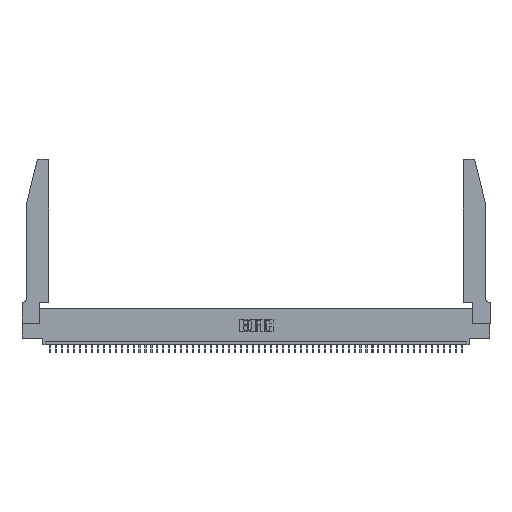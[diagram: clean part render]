
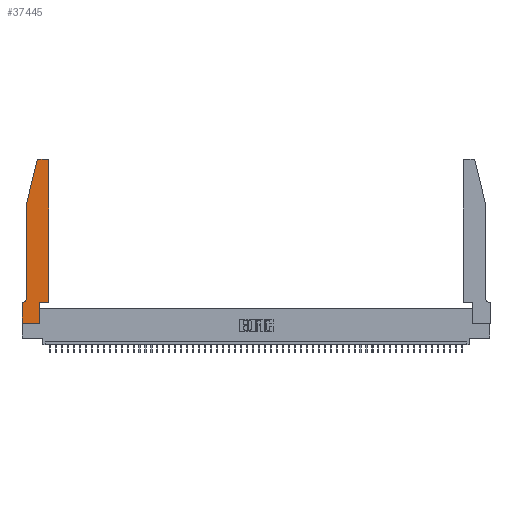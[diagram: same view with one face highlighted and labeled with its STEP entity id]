
A CAD part, top view. The second image highlights one B-rep face of the part: STEP entity #37445.
In plain terms, the highlighted planar face has unit normal (0, 0, 1).
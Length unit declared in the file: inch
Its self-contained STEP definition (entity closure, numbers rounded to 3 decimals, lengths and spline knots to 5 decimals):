
#258 = ORIENTED_EDGE ( 'NONE', *, *, #11909, .T. ) ;
#563 = CARTESIAN_POINT ( 'NONE',  ( 0., 0., 0.37 ) ) ;
#596 = VECTOR ( 'NONE', #46374, 39.37008 ) ;
#936 = VERTEX_POINT ( 'NONE', #29990 ) ;
#1106 = CARTESIAN_POINT ( 'NONE',  ( 0.0755, 2., 0.37 ) ) ;
#1564 = CARTESIAN_POINT ( 'NONE',  ( 0.4505, 0.35, 0.37 ) ) ;
#2447 = CIRCLE ( 'NONE', #44126, 0.03 ) ;
#2887 = VERTEX_POINT ( 'NONE', #3976 ) ;
#3383 = VERTEX_POINT ( 'NONE', #29261 ) ;
#3976 = CARTESIAN_POINT ( 'NONE',  ( 0.4205, 2.75, 0.37 ) ) ;
#4281 = ORIENTED_EDGE ( 'NONE', *, *, #52299, .T. ) ;
#6387 = CARTESIAN_POINT ( 'NONE',  ( 0.0755, 2., 0.37 ) ) ;
#6652 = VECTOR ( 'NONE', #6730, 39.37008 ) ;
#6730 = DIRECTION ( 'NONE',  ( 0., -1., 0. ) ) ;
#6797 = DIRECTION ( 'NONE',  ( 0., 0., 1. ) ) ;
#7917 = DIRECTION ( 'NONE',  ( -1., 0., 0. ) ) ;
#8159 = CARTESIAN_POINT ( 'NONE',  ( 0., 0.35, 0.37 ) ) ;
#8361 = VERTEX_POINT ( 'NONE', #37701 ) ;
#8521 = VECTOR ( 'NONE', #18210, 39.37008 ) ;
#9204 = LINE ( 'NONE', #1564, #8521 ) ;
#9491 = EDGE_CURVE ( 'NONE', #39485, #41257, #18701, .T. ) ;
#9911 = PLANE ( 'NONE',  #30217 ) ;
#10360 = LINE ( 'NONE', #26159, #34873 ) ;
#10808 = CARTESIAN_POINT ( 'NONE',  ( 0.2865, 0.35, 0.37 ) ) ;
#11101 = VECTOR ( 'NONE', #22383, 39.37008 ) ;
#11566 = ORIENTED_EDGE ( 'NONE', *, *, #42108, .T. ) ;
#11909 = EDGE_CURVE ( 'NONE', #45939, #35143, #14349, .T. ) ;
#12085 = AXIS2_PLACEMENT_3D ( 'NONE', #32163, #6797, #15284 ) ;
#12240 = CARTESIAN_POINT ( 'NONE',  ( 0.0055, 0.35, 0.37 ) ) ;
#12874 = VERTEX_POINT ( 'NONE', #18294 ) ;
#12935 = CIRCLE ( 'NONE', #12085, 0.03 ) ;
#14283 = DIRECTION ( 'NONE',  ( 0., 0., 1. ) ) ;
#14349 = LINE ( 'NONE', #17869, #30030 ) ;
#15284 = DIRECTION ( 'NONE',  ( 1., 0., 0. ) ) ;
#16273 = EDGE_LOOP ( 'NONE', ( #22857, #35106, #39636, #48043, #29615, #33045, #4281, #258, #11566, #48635, #43502, #42557 ) ) ;
#17751 = LINE ( 'NONE', #563, #596 ) ;
#17869 = CARTESIAN_POINT ( 'NONE',  ( 0., 0., 0.37 ) ) ;
#18210 = DIRECTION ( 'NONE',  ( 0., 1., 0. ) ) ;
#18294 = CARTESIAN_POINT ( 'NONE',  ( 0.25487, 2.72718, 0.37 ) ) ;
#18701 = CIRCLE ( 'NONE', #34368, 0.07 ) ;
#19754 = EDGE_CURVE ( 'NONE', #25671, #3383, #10360, .T. ) ;
#21953 = LINE ( 'NONE', #6387, #46335 ) ;
#21958 = EDGE_CURVE ( 'NONE', #12874, #46717, #21953, .T. ) ;
#22383 = DIRECTION ( 'NONE',  ( -1., 0., 0. ) ) ;
#22506 = DIRECTION ( 'NONE',  ( 1., 0., 0. ) ) ;
#22708 = CARTESIAN_POINT ( 'NONE',  ( 0.0055, 0.42, 0.37 ) ) ;
#22857 = ORIENTED_EDGE ( 'NONE', *, *, #52084, .T. ) ;
#23957 = EDGE_CURVE ( 'NONE', #46717, #39485, #47458, .T. ) ;
#25671 = VERTEX_POINT ( 'NONE', #10808 ) ;
#26159 = CARTESIAN_POINT ( 'NONE',  ( 0.4505, 0.35, 0.37 ) ) ;
#27401 = CARTESIAN_POINT ( 'NONE',  ( 0.284, 2.72, 0.37 ) ) ;
#28149 = VERTEX_POINT ( 'NONE', #8159 ) ;
#28371 = DIRECTION ( 'NONE',  ( 0., 0., -1. ) ) ;
#29261 = CARTESIAN_POINT ( 'NONE',  ( 0.4505, 0.35, 0.37 ) ) ;
#29615 = ORIENTED_EDGE ( 'NONE', *, *, #9491, .T. ) ;
#29990 = CARTESIAN_POINT ( 'NONE',  ( 0.4505, 2.72, 0.37 ) ) ;
#30030 = VECTOR ( 'NONE', #22506, 39.37008 ) ;
#30208 = CARTESIAN_POINT ( 'NONE',  ( 0.0755, 0.42, 0.37 ) ) ;
#30217 = AXIS2_PLACEMENT_3D ( 'NONE', #43148, #14283, #30877 ) ;
#30592 = CARTESIAN_POINT ( 'NONE',  ( 0., 0., 0.37 ) ) ;
#30810 = LINE ( 'NONE', #51836, #11101 ) ;
#30877 = DIRECTION ( 'NONE',  ( 1., 0., 0. ) ) ;
#30942 = CARTESIAN_POINT ( 'NONE',  ( 0.2865, 0.35, 0.37 ) ) ;
#31762 = DIRECTION ( 'NONE',  ( 1., 0., 0. ) ) ;
#32163 = CARTESIAN_POINT ( 'NONE',  ( 0.4205, 2.72, 0.37 ) ) ;
#32829 = VECTOR ( 'NONE', #47264, 39.37008 ) ;
#33045 = ORIENTED_EDGE ( 'NONE', *, *, #52415, .T. ) ;
#34368 = AXIS2_PLACEMENT_3D ( 'NONE', #22708, #28371, #7917 ) ;
#34873 = VECTOR ( 'NONE', #38696, 39.37008 ) ;
#35106 = ORIENTED_EDGE ( 'NONE', *, *, #51740, .T. ) ;
#35143 = VERTEX_POINT ( 'NONE', #50332 ) ;
#35266 = CARTESIAN_POINT ( 'NONE',  ( 0.2605, 2.75, 0.37 ) ) ;
#35871 = DIRECTION ( 'NONE',  ( 0., 0., 1. ) ) ;
#37445 = ADVANCED_FACE ( 'NONE', ( #47255 ), #9911, .T. ) ;
#37701 = CARTESIAN_POINT ( 'NONE',  ( 0.284, 2.75, 0.37 ) ) ;
#38696 = DIRECTION ( 'NONE',  ( 1., 0., 0. ) ) ;
#39485 = VERTEX_POINT ( 'NONE', #30208 ) ;
#39636 = ORIENTED_EDGE ( 'NONE', *, *, #21958, .T. ) ;
#40513 = EDGE_CURVE ( 'NONE', #3383, #936, #9204, .T. ) ;
#41180 = EDGE_CURVE ( 'NONE', #936, #2887, #12935, .T. ) ;
#41257 = VERTEX_POINT ( 'NONE', #12240 ) ;
#42108 = EDGE_CURVE ( 'NONE', #35143, #25671, #43764, .T. ) ;
#42557 = ORIENTED_EDGE ( 'NONE', *, *, #41180, .T. ) ;
#43148 = CARTESIAN_POINT ( 'NONE',  ( 0., 0.35, 0.37 ) ) ;
#43502 = ORIENTED_EDGE ( 'NONE', *, *, #40513, .T. ) ;
#43764 = LINE ( 'NONE', #30942, #52247 ) ;
#43974 = LINE ( 'NONE', #35266, #32829 ) ;
#44126 = AXIS2_PLACEMENT_3D ( 'NONE', #27401, #35871, #31762 ) ;
#45939 = VERTEX_POINT ( 'NONE', #30592 ) ;
#46335 = VECTOR ( 'NONE', #51125, 39.37008 ) ;
#46374 = DIRECTION ( 'NONE',  ( 0., -1., 0. ) ) ;
#46717 = VERTEX_POINT ( 'NONE', #50938 ) ;
#47255 = FACE_OUTER_BOUND ( 'NONE', #16273, .T. ) ;
#47264 = DIRECTION ( 'NONE',  ( -1., 0., 0. ) ) ;
#47458 = LINE ( 'NONE', #1106, #6652 ) ;
#47587 = DIRECTION ( 'NONE',  ( 0., 1., 0. ) ) ;
#48043 = ORIENTED_EDGE ( 'NONE', *, *, #23957, .T. ) ;
#48635 = ORIENTED_EDGE ( 'NONE', *, *, #19754, .T. ) ;
#50332 = CARTESIAN_POINT ( 'NONE',  ( 0.2865, 0., 0.37 ) ) ;
#50938 = CARTESIAN_POINT ( 'NONE',  ( 0.0755, 2., 0.37 ) ) ;
#51125 = DIRECTION ( 'NONE',  ( -0.239, -0.971, 0. ) ) ;
#51740 = EDGE_CURVE ( 'NONE', #8361, #12874, #2447, .T. ) ;
#51836 = CARTESIAN_POINT ( 'NONE',  ( 0.0755, 0.35, 0.37 ) ) ;
#52084 = EDGE_CURVE ( 'NONE', #2887, #8361, #43974, .T. ) ;
#52247 = VECTOR ( 'NONE', #47587, 39.37008 ) ;
#52299 = EDGE_CURVE ( 'NONE', #28149, #45939, #17751, .T. ) ;
#52415 = EDGE_CURVE ( 'NONE', #41257, #28149, #30810, .T. ) ;
